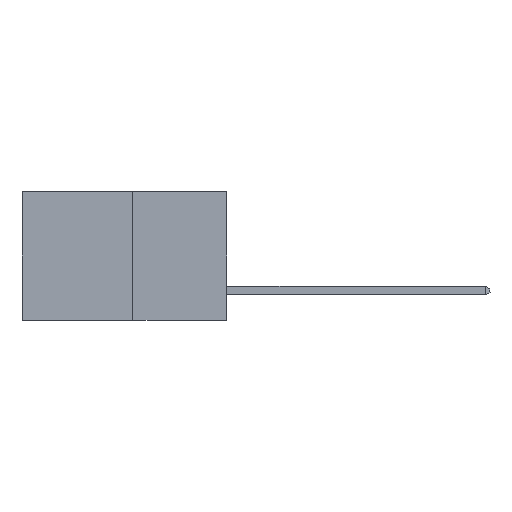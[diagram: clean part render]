
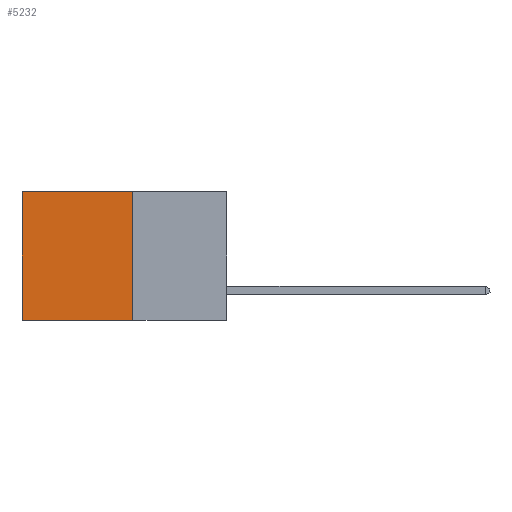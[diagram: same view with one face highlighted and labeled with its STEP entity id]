
A CAD part, left-side view. The second image highlights one B-rep face of the part: STEP entity #5232.
In plain terms, the highlighted planar face has unit normal (-1, 0, 0).
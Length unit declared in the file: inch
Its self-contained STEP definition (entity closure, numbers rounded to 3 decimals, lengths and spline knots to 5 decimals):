
#577 = CARTESIAN_POINT ( 'NONE',  ( 0.277, 0.27, -0.37 ) ) ;
#684 = ORIENTED_EDGE ( 'NONE', *, *, #4026, .T. ) ;
#930 = AXIS2_PLACEMENT_3D ( 'NONE', #7343, #6757, #6727 ) ;
#965 = DIRECTION ( 'NONE',  ( 0., 0., -1. ) ) ;
#986 = CARTESIAN_POINT ( 'NONE',  ( 0.277, 0.27, -0.37 ) ) ;
#1044 = ORIENTED_EDGE ( 'NONE', *, *, #7956, .T. ) ;
#1544 = CARTESIAN_POINT ( 'NONE',  ( 0.277, 0.27, 0. ) ) ;
#1616 = EDGE_CURVE ( 'NONE', #5636, #4320, #6153, .T. ) ;
#2503 = LINE ( 'NONE', #986, #7252 ) ;
#2660 = EDGE_CURVE ( 'NONE', #5340, #5636, #2503, .T. ) ;
#2770 = CARTESIAN_POINT ( 'NONE',  ( 0.277, 0.59, 0. ) ) ;
#3133 = VERTEX_POINT ( 'NONE', #2770 ) ;
#3139 = VECTOR ( 'NONE', #7550, 39.37008 ) ;
#3877 = ORIENTED_EDGE ( 'NONE', *, *, #2660, .F. ) ;
#3901 = EDGE_LOOP ( 'NONE', ( #684, #7379, #3877, #1044 ) ) ;
#3911 = DIRECTION ( 'NONE',  ( 0., 1., 0. ) ) ;
#4026 = EDGE_CURVE ( 'NONE', #3133, #4320, #7896, .T. ) ;
#4120 = VECTOR ( 'NONE', #3911, 39.37008 ) ;
#4261 = CARTESIAN_POINT ( 'NONE',  ( 0.277, 0.59, -0.37 ) ) ;
#4320 = VERTEX_POINT ( 'NONE', #4261 ) ;
#5232 = ADVANCED_FACE ( 'NONE', ( #7132 ), #6640, .F. ) ;
#5322 = DIRECTION ( 'NONE',  ( 0., 1., 0. ) ) ;
#5340 = VERTEX_POINT ( 'NONE', #1544 ) ;
#5636 = VERTEX_POINT ( 'NONE', #577 ) ;
#6153 = LINE ( 'NONE', #7727, #7764 ) ;
#6640 = PLANE ( 'NONE',  #930 ) ;
#6727 = DIRECTION ( 'NONE',  ( 0., 0., -1. ) ) ;
#6757 = DIRECTION ( 'NONE',  ( 1., 0., 0. ) ) ;
#7132 = FACE_OUTER_BOUND ( 'NONE', #3901, .T. ) ;
#7246 = LINE ( 'NONE', #7979, #4120 ) ;
#7252 = VECTOR ( 'NONE', #965, 39.37008 ) ;
#7343 = CARTESIAN_POINT ( 'NONE',  ( 0.277, 0.27, -0.37 ) ) ;
#7347 = CARTESIAN_POINT ( 'NONE',  ( 0.277, 0.59, -0.37 ) ) ;
#7379 = ORIENTED_EDGE ( 'NONE', *, *, #1616, .F. ) ;
#7550 = DIRECTION ( 'NONE',  ( 0., 0., -1. ) ) ;
#7727 = CARTESIAN_POINT ( 'NONE',  ( 0.277, 0.27, -0.37 ) ) ;
#7764 = VECTOR ( 'NONE', #5322, 39.37008 ) ;
#7896 = LINE ( 'NONE', #7347, #3139 ) ;
#7956 = EDGE_CURVE ( 'NONE', #5340, #3133, #7246, .T. ) ;
#7979 = CARTESIAN_POINT ( 'NONE',  ( 0.277, 0.27, 0. ) ) ;
